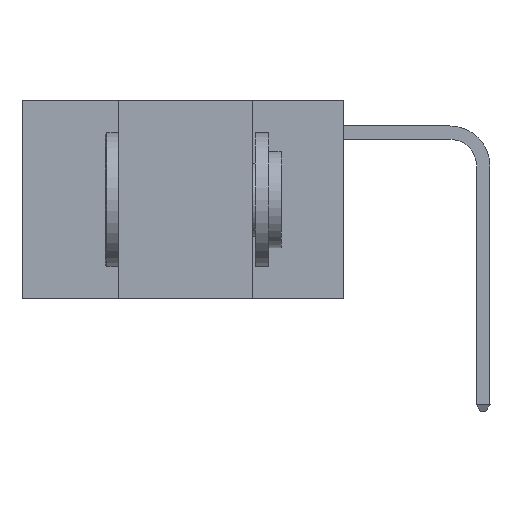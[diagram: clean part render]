
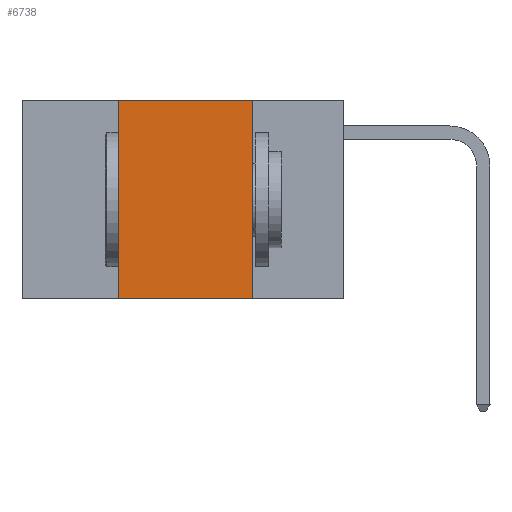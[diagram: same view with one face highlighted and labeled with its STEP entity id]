
A CAD part, left-side view. The second image highlights one B-rep face of the part: STEP entity #6738.
In plain terms, the highlighted planar face has unit normal (-1, 0, 0).
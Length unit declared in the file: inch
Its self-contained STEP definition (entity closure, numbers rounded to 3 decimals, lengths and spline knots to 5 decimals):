
#302 = AXIS2_PLACEMENT_3D ( 'NONE', #8267, #7539, #2030 ) ;
#1150 = EDGE_CURVE ( 'NONE', #6473, #7004, #6607, .T. ) ;
#1705 = CARTESIAN_POINT ( 'NONE',  ( 0., 0.6, -0.37 ) ) ;
#1784 = EDGE_CURVE ( 'NONE', #6473, #4787, #7024, .T. ) ;
#2030 = DIRECTION ( 'NONE',  ( 0., 0., -1. ) ) ;
#2095 = VECTOR ( 'NONE', #6283, 39.37008 ) ;
#2248 = DIRECTION ( 'NONE',  ( 0., -1., 0. ) ) ;
#2253 = VECTOR ( 'NONE', #2248, 39.37008 ) ;
#2417 = EDGE_CURVE ( 'NONE', #6298, #7004, #10922, .T. ) ;
#2676 = LINE ( 'NONE', #7072, #7284 ) ;
#4787 = VERTEX_POINT ( 'NONE', #6514 ) ;
#5687 = DIRECTION ( 'NONE',  ( 0., 0., -1. ) ) ;
#6283 = DIRECTION ( 'NONE',  ( 0., 0., 1. ) ) ;
#6298 = VERTEX_POINT ( 'NONE', #10915 ) ;
#6441 = ORIENTED_EDGE ( 'NONE', *, *, #2417, .F. ) ;
#6452 = ORIENTED_EDGE ( 'NONE', *, *, #7706, .F. ) ;
#6473 = VERTEX_POINT ( 'NONE', #10338 ) ;
#6514 = CARTESIAN_POINT ( 'NONE',  ( 0., 0.42, 0. ) ) ;
#6607 = LINE ( 'NONE', #1705, #2253 ) ;
#6738 = ADVANCED_FACE ( 'NONE', ( #10708 ), #10689, .F. ) ;
#6910 = ORIENTED_EDGE ( 'NONE', *, *, #1784, .F. ) ;
#7004 = VERTEX_POINT ( 'NONE', #7886 ) ;
#7024 = LINE ( 'NONE', #9127, #2095 ) ;
#7072 = CARTESIAN_POINT ( 'NONE',  ( 0., 0.6, 0. ) ) ;
#7080 = ORIENTED_EDGE ( 'NONE', *, *, #1150, .T. ) ;
#7284 = VECTOR ( 'NONE', #7911, 39.37008 ) ;
#7539 = DIRECTION ( 'NONE',  ( 1., 0., 0. ) ) ;
#7706 = EDGE_CURVE ( 'NONE', #4787, #6298, #2676, .T. ) ;
#7886 = CARTESIAN_POINT ( 'NONE',  ( 0., 0.17, -0.37 ) ) ;
#7911 = DIRECTION ( 'NONE',  ( 0., -1., 0. ) ) ;
#8267 = CARTESIAN_POINT ( 'NONE',  ( 0., 0.6, 0. ) ) ;
#8411 = EDGE_LOOP ( 'NONE', ( #6441, #6452, #6910, #7080 ) ) ;
#8770 = VECTOR ( 'NONE', #5687, 39.37008 ) ;
#9058 = CARTESIAN_POINT ( 'NONE',  ( 0., 0.17, 0. ) ) ;
#9127 = CARTESIAN_POINT ( 'NONE',  ( 0., 0.42, 0. ) ) ;
#10338 = CARTESIAN_POINT ( 'NONE',  ( 0., 0.42, -0.37 ) ) ;
#10689 = PLANE ( 'NONE',  #302 ) ;
#10708 = FACE_OUTER_BOUND ( 'NONE', #8411, .T. ) ;
#10915 = CARTESIAN_POINT ( 'NONE',  ( 0., 0.17, 0. ) ) ;
#10922 = LINE ( 'NONE', #9058, #8770 ) ;
